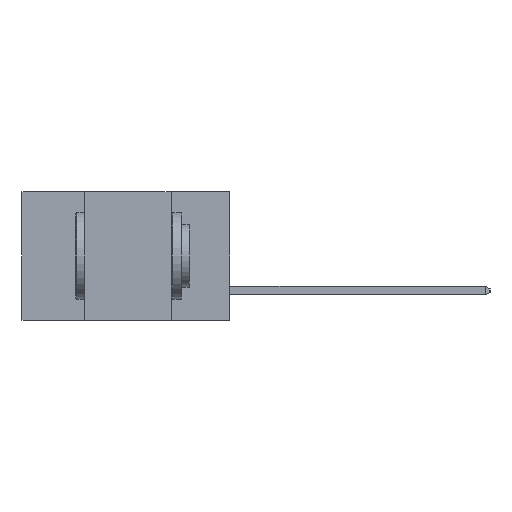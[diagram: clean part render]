
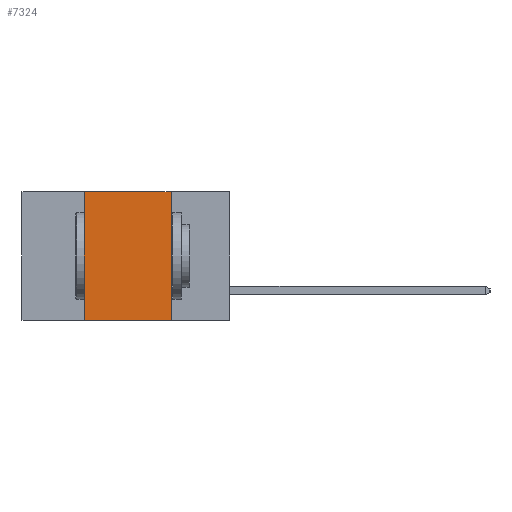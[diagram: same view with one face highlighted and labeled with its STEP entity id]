
A CAD part, left-side view. The second image highlights one B-rep face of the part: STEP entity #7324.
In plain terms, the highlighted planar face has unit normal (-1, 0, 0).
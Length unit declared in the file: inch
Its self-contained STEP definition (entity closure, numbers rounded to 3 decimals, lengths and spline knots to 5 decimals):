
#13 = EDGE_LOOP ( 'NONE', ( #3270, #274, #694, #3484 ) ) ;
#21 = VECTOR ( 'NONE', #7269, 39.37008 ) ;
#203 = LINE ( 'NONE', #4144, #2232 ) ;
#263 = EDGE_CURVE ( 'NONE', #2362, #6883, #544, .T. ) ;
#271 = LINE ( 'NONE', #2186, #21 ) ;
#274 = ORIENTED_EDGE ( 'NONE', *, *, #1255, .F. ) ;
#544 = LINE ( 'NONE', #7160, #2080 ) ;
#694 = ORIENTED_EDGE ( 'NONE', *, *, #263, .F. ) ;
#978 = LINE ( 'NONE', #9160, #8734 ) ;
#1255 = EDGE_CURVE ( 'NONE', #6883, #6754, #978, .T. ) ;
#1350 = PLANE ( 'NONE',  #5904 ) ;
#1877 = DIRECTION ( 'NONE',  ( 0., 0., -1. ) ) ;
#2080 = VECTOR ( 'NONE', #8352, 39.37008 ) ;
#2186 = CARTESIAN_POINT ( 'NONE',  ( 0., 0.6, -0.37 ) ) ;
#2232 = VECTOR ( 'NONE', #1877, 39.37008 ) ;
#2362 = VERTEX_POINT ( 'NONE', #8456 ) ;
#2942 = DIRECTION ( 'NONE',  ( 0., 0., -1. ) ) ;
#3270 = ORIENTED_EDGE ( 'NONE', *, *, #5304, .F. ) ;
#3362 = VERTEX_POINT ( 'NONE', #8784 ) ;
#3484 = ORIENTED_EDGE ( 'NONE', *, *, #7355, .T. ) ;
#4144 = CARTESIAN_POINT ( 'NONE',  ( 0., 0.17, -0.37 ) ) ;
#5031 = DIRECTION ( 'NONE',  ( 0., -1., 0. ) ) ;
#5304 = EDGE_CURVE ( 'NONE', #6754, #3362, #203, .T. ) ;
#5328 = CARTESIAN_POINT ( 'NONE',  ( 0., 0.42, 0. ) ) ;
#5904 = AXIS2_PLACEMENT_3D ( 'NONE', #6565, #7238, #2942 ) ;
#6451 = FACE_OUTER_BOUND ( 'NONE', #13, .T. ) ;
#6565 = CARTESIAN_POINT ( 'NONE',  ( 0., 0.6, 0. ) ) ;
#6754 = VERTEX_POINT ( 'NONE', #9362 ) ;
#6883 = VERTEX_POINT ( 'NONE', #5328 ) ;
#7160 = CARTESIAN_POINT ( 'NONE',  ( 0., 0.42, -0.37 ) ) ;
#7238 = DIRECTION ( 'NONE',  ( 1., 0., 0. ) ) ;
#7269 = DIRECTION ( 'NONE',  ( 0., -1., 0. ) ) ;
#7324 = ADVANCED_FACE ( 'NONE', ( #6451 ), #1350, .F. ) ;
#7355 = EDGE_CURVE ( 'NONE', #2362, #3362, #271, .T. ) ;
#8352 = DIRECTION ( 'NONE',  ( 0., 0., 1. ) ) ;
#8456 = CARTESIAN_POINT ( 'NONE',  ( 0., 0.42, -0.37 ) ) ;
#8734 = VECTOR ( 'NONE', #5031, 39.37008 ) ;
#8784 = CARTESIAN_POINT ( 'NONE',  ( 0., 0.17, -0.37 ) ) ;
#9160 = CARTESIAN_POINT ( 'NONE',  ( 0., 0.6, 0. ) ) ;
#9362 = CARTESIAN_POINT ( 'NONE',  ( 0., 0.17, 0. ) ) ;
